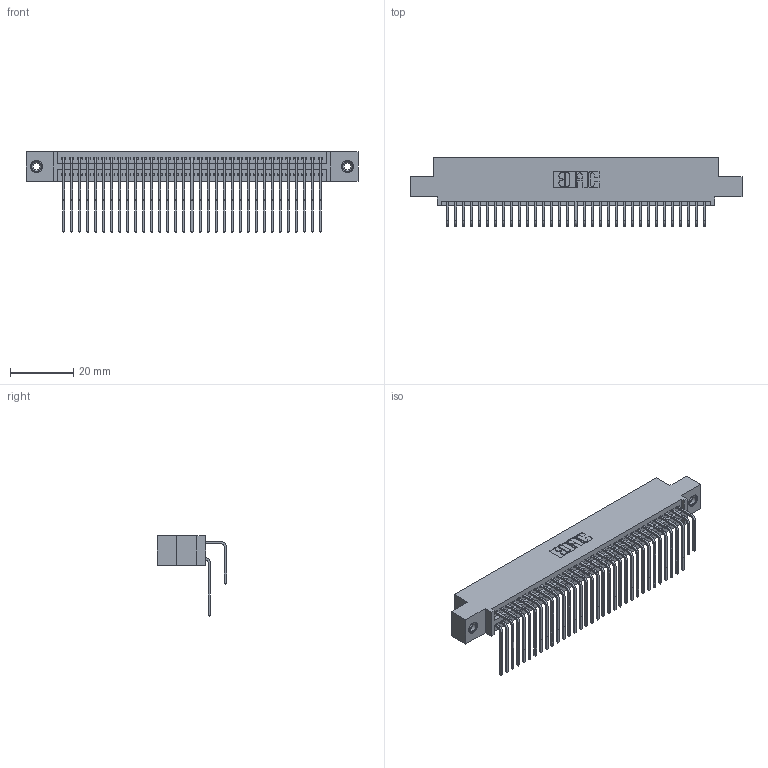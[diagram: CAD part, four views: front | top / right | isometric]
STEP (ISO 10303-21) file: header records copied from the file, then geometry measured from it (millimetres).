
FILE_DESCRIPTION (( 'STEP AP203' ), '1' );
FILE_NAME ('345-066-558-508.STEP', '2019-10-30T18:26:43', ( '' ), ( '' ), 'SwSTEP 2.0', 'SolidWorks 2016', '' );
FILE_SCHEMA (( 'CONFIG_CONTROL_DESIGN' ));
Length unit declared in the file: inch
Products named in the file (5): 345-066-558-508; 345-292-001_558 559 Tail - 1; 345 Part_0.110 Offset - 0.156 Dia-TI; 345-292-001_558 Tail - 2; 345-250-001_345-250-003-102
Assembly tree (69 placements, depth 2):
  345-066-558-508
    345 Part_0.110 Offset - 0.156 Dia-TI
    345-292-001_558 559 Tail - 1  x33
    345-292-001_558 Tail - 2  x33
    345-250-001_345-250-003-102  x2
Bounding box: 105.03 x 21.83 x 25.53 mm (x, y, z)
Volume: 10419.9 mm3; surface area: 17124.7 mm2
Topology: 69 solids, 69 shells, 3622 faces, 10719 edges, 7050 vertices
Faces by surface type: plane 2426, cylinder 1180, cone 12, torus 4
Entity records: 30074 total; most frequent: CARTESIAN_POINT 5078, ORIENTED_EDGE 4954, DIRECTION 4487, EDGE_CURVE 2477, LINE 2153, VECTOR 2153, VERTEX_POINT 1644, AXIS2_PLACEMENT_3D 1167
